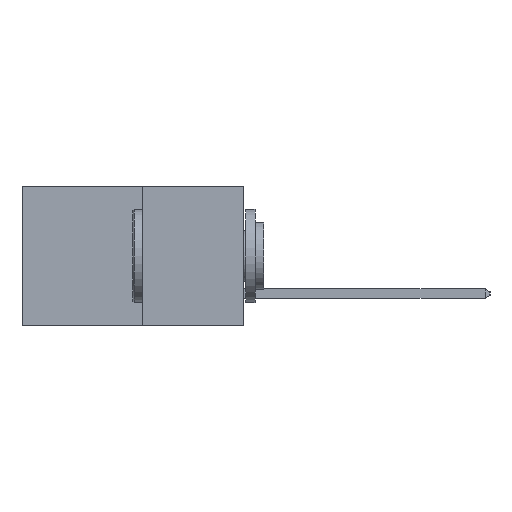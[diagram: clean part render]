
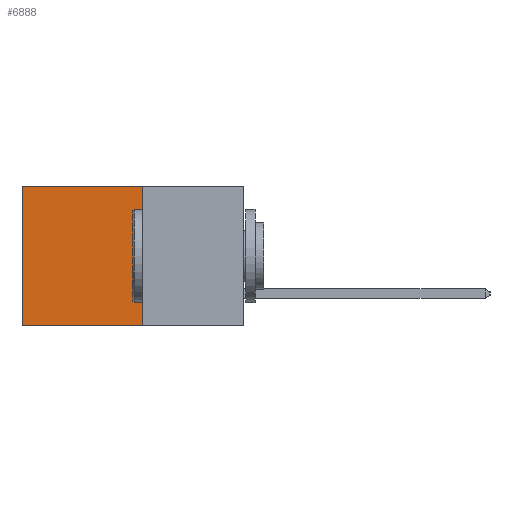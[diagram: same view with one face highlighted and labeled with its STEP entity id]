
A CAD part, left-side view. The second image highlights one B-rep face of the part: STEP entity #6888.
In plain terms, the highlighted planar face has unit normal (-1, 0, 0).
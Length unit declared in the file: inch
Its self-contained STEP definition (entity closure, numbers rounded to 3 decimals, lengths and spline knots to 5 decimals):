
#851 = VERTEX_POINT ( 'NONE', #8105 ) ;
#1475 = VERTEX_POINT ( 'NONE', #23876 ) ;
#2216 = CARTESIAN_POINT ( 'NONE',  ( 0.277, 0.27, -0.37 ) ) ;
#2405 = VECTOR ( 'NONE', #19977, 39.37008 ) ;
#3215 = PLANE ( 'NONE',  #12916 ) ;
#3310 = DIRECTION ( 'NONE',  ( 1., 0., 0. ) ) ;
#5107 = EDGE_CURVE ( 'NONE', #851, #20837, #11937, .T. ) ;
#5193 = FACE_OUTER_BOUND ( 'NONE', #11773, .T. ) ;
#6212 = CARTESIAN_POINT ( 'NONE',  ( 0.277, 0.27, -0.37 ) ) ;
#6238 = ORIENTED_EDGE ( 'NONE', *, *, #14174, .T. ) ;
#6499 = VERTEX_POINT ( 'NONE', #10897 ) ;
#6644 = DIRECTION ( 'NONE',  ( 0., 0., -1. ) ) ;
#6888 = ADVANCED_FACE ( 'NONE', ( #5193 ), #3215, .F. ) ;
#7712 = LINE ( 'NONE', #2216, #2405 ) ;
#8105 = CARTESIAN_POINT ( 'NONE',  ( 0.277, 0.27, 0. ) ) ;
#10897 = CARTESIAN_POINT ( 'NONE',  ( 0.277, 0.59, 0. ) ) ;
#11773 = EDGE_LOOP ( 'NONE', ( #6238, #15666, #18561, #27697 ) ) ;
#11937 = LINE ( 'NONE', #6212, #22662 ) ;
#12702 = CARTESIAN_POINT ( 'NONE',  ( 0.277, 0.59, -0.37 ) ) ;
#12916 = AXIS2_PLACEMENT_3D ( 'NONE', #14484, #3310, #18853 ) ;
#13403 = CARTESIAN_POINT ( 'NONE',  ( 0.277, 0.27, -0.37 ) ) ;
#14174 = EDGE_CURVE ( 'NONE', #6499, #1475, #25708, .T. ) ;
#14484 = CARTESIAN_POINT ( 'NONE',  ( 0.277, 0.27, -0.37 ) ) ;
#15666 = ORIENTED_EDGE ( 'NONE', *, *, #27498, .F. ) ;
#17932 = LINE ( 'NONE', #22388, #23013 ) ;
#18561 = ORIENTED_EDGE ( 'NONE', *, *, #5107, .F. ) ;
#18853 = DIRECTION ( 'NONE',  ( 0., 0., -1. ) ) ;
#19913 = VECTOR ( 'NONE', #25781, 39.37008 ) ;
#19977 = DIRECTION ( 'NONE',  ( 0., 1., 0. ) ) ;
#20837 = VERTEX_POINT ( 'NONE', #13403 ) ;
#21564 = EDGE_CURVE ( 'NONE', #851, #6499, #17932, .T. ) ;
#22388 = CARTESIAN_POINT ( 'NONE',  ( 0.277, 0.27, 0. ) ) ;
#22662 = VECTOR ( 'NONE', #6644, 39.37008 ) ;
#23013 = VECTOR ( 'NONE', #24600, 39.37008 ) ;
#23876 = CARTESIAN_POINT ( 'NONE',  ( 0.277, 0.59, -0.37 ) ) ;
#24600 = DIRECTION ( 'NONE',  ( 0., 1., 0. ) ) ;
#25708 = LINE ( 'NONE', #12702, #19913 ) ;
#25781 = DIRECTION ( 'NONE',  ( 0., 0., -1. ) ) ;
#27498 = EDGE_CURVE ( 'NONE', #20837, #1475, #7712, .T. ) ;
#27697 = ORIENTED_EDGE ( 'NONE', *, *, #21564, .T. ) ;
